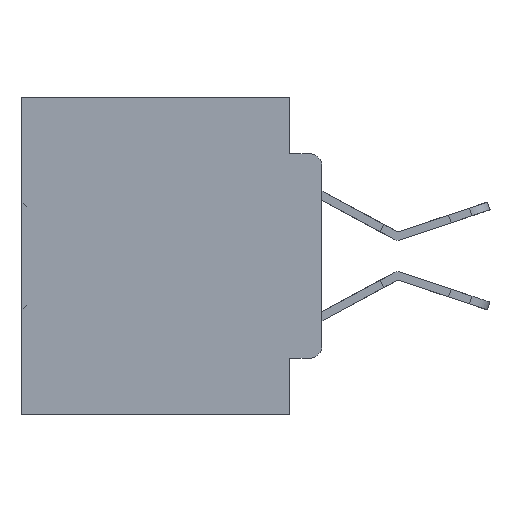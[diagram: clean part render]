
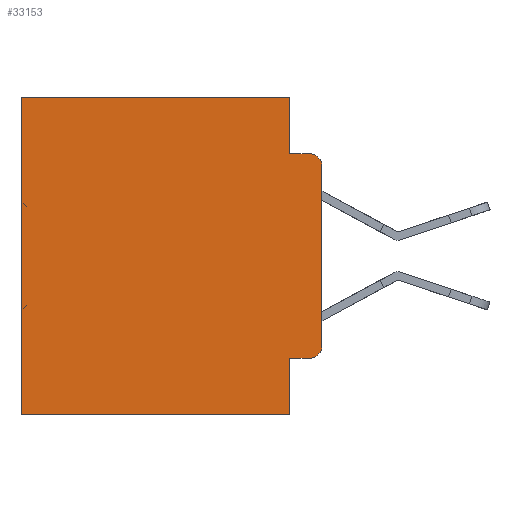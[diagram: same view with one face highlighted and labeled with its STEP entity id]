
A CAD part, left-side view. The second image highlights one B-rep face of the part: STEP entity #33153.
In plain terms, the highlighted planar face has unit normal (-1, 0, 0).
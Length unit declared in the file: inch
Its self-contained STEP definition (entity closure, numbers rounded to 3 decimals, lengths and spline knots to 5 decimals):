
#125 = DIRECTION ( 'NONE',  ( 0., 0., -1. ) ) ;
#1004 = EDGE_CURVE ( 'NONE', #16473, #6473, #36695, .T. ) ;
#1269 = DIRECTION ( 'NONE',  ( 0., 0., -1. ) ) ;
#2205 = PLANE ( 'NONE',  #34444 ) ;
#2926 = CARTESIAN_POINT ( 'NONE',  ( 0.298, 0., 0. ) ) ;
#4104 = DIRECTION ( 'NONE',  ( 0., 0., -1. ) ) ;
#4552 = ORIENTED_EDGE ( 'NONE', *, *, #5437, .T. ) ;
#4838 = CARTESIAN_POINT ( 'NONE',  ( 0.298, 0.051, 0. ) ) ;
#5370 = CARTESIAN_POINT ( 'NONE',  ( 0.298, 0.051, -0.4115 ) ) ;
#5437 = EDGE_CURVE ( 'NONE', #27533, #5798, #13555, .T. ) ;
#5631 = ORIENTED_EDGE ( 'NONE', *, *, #1004, .F. ) ;
#5798 = VERTEX_POINT ( 'NONE', #19166 ) ;
#6473 = VERTEX_POINT ( 'NONE', #28445 ) ;
#6567 = VECTOR ( 'NONE', #1269, 39.37008 ) ;
#7420 = AXIS2_PLACEMENT_3D ( 'NONE', #29748, #24130, #18164 ) ;
#8369 = VECTOR ( 'NONE', #14252, 39.37008 ) ;
#8525 = DIRECTION ( 'NONE',  ( 0., 0., -1. ) ) ;
#8700 = DIRECTION ( 'NONE',  ( -1., 0., 0. ) ) ;
#8850 = ORIENTED_EDGE ( 'NONE', *, *, #24724, .T. ) ;
#9277 = EDGE_CURVE ( 'NONE', #29825, #14734, #18212, .T. ) ;
#9358 = DIRECTION ( 'NONE',  ( 0., 1., 0. ) ) ;
#9427 = CARTESIAN_POINT ( 'NONE',  ( 0.298, 0., -0.3915 ) ) ;
#9529 = EDGE_CURVE ( 'NONE', #6473, #16681, #23020, .T. ) ;
#10790 = LINE ( 'NONE', #4838, #31050 ) ;
#10840 = CARTESIAN_POINT ( 'NONE',  ( 0.298, 0.473, 0. ) ) ;
#10865 = EDGE_CURVE ( 'NONE', #32376, #20447, #12300, .T. ) ;
#10897 = VECTOR ( 'NONE', #33511, 39.37008 ) ;
#11556 = CIRCLE ( 'NONE', #7420, 0.02 ) ;
#11945 = CARTESIAN_POINT ( 'NONE',  ( 0.298, 0.473, -0.5 ) ) ;
#12163 = ORIENTED_EDGE ( 'NONE', *, *, #10865, .T. ) ;
#12300 = LINE ( 'NONE', #32654, #34696 ) ;
#13555 = LINE ( 'NONE', #24939, #27891 ) ;
#14252 = DIRECTION ( 'NONE',  ( 0., -1., 0. ) ) ;
#14734 = VERTEX_POINT ( 'NONE', #9427 ) ;
#15325 = CARTESIAN_POINT ( 'NONE',  ( 0.298, 0., -0.5 ) ) ;
#15423 = CARTESIAN_POINT ( 'NONE',  ( 0.298, 0., 0. ) ) ;
#15704 = VECTOR ( 'NONE', #30556, 39.37008 ) ;
#16250 = ORIENTED_EDGE ( 'NONE', *, *, #9277, .F. ) ;
#16473 = VERTEX_POINT ( 'NONE', #17217 ) ;
#16674 = LINE ( 'NONE', #24885, #10897 ) ;
#16681 = VERTEX_POINT ( 'NONE', #23570 ) ;
#16903 = CARTESIAN_POINT ( 'NONE',  ( 0.298, 0.051, 0. ) ) ;
#17217 = CARTESIAN_POINT ( 'NONE',  ( 0.298, 0.051, 0. ) ) ;
#17577 = ORIENTED_EDGE ( 'NONE', *, *, #19497, .F. ) ;
#18164 = DIRECTION ( 'NONE',  ( 0., 0., -1. ) ) ;
#18212 = LINE ( 'NONE', #15423, #6567 ) ;
#19030 = ORIENTED_EDGE ( 'NONE', *, *, #25948, .T. ) ;
#19166 = CARTESIAN_POINT ( 'NONE',  ( 0.298, 0.02, -0.4115 ) ) ;
#19497 = EDGE_CURVE ( 'NONE', #27533, #29347, #10790, .T. ) ;
#19710 = DIRECTION ( 'NONE',  ( 0., -1., 0. ) ) ;
#19778 = ORIENTED_EDGE ( 'NONE', *, *, #36129, .F. ) ;
#19885 = FACE_OUTER_BOUND ( 'NONE', #29119, .T. ) ;
#19973 = AXIS2_PLACEMENT_3D ( 'NONE', #23063, #8700, #8525 ) ;
#20447 = VERTEX_POINT ( 'NONE', #11945 ) ;
#21294 = ORIENTED_EDGE ( 'NONE', *, *, #9529, .F. ) ;
#23020 = LINE ( 'NONE', #28456, #8369 ) ;
#23063 = CARTESIAN_POINT ( 'NONE',  ( 0.298, 0.02, -0.3915 ) ) ;
#23203 = EDGE_CURVE ( 'NONE', #16473, #32376, #16674, .T. ) ;
#23352 = LINE ( 'NONE', #15325, #23844 ) ;
#23550 = CIRCLE ( 'NONE', #19973, 0.02 ) ;
#23570 = CARTESIAN_POINT ( 'NONE',  ( 0.298, 0.02, -0.0885 ) ) ;
#23844 = VECTOR ( 'NONE', #9358, 39.37008 ) ;
#24130 = DIRECTION ( 'NONE',  ( -1., 0., 0. ) ) ;
#24724 = EDGE_CURVE ( 'NONE', #29825, #16681, #11556, .T. ) ;
#24885 = CARTESIAN_POINT ( 'NONE',  ( 0.298, 0., 0. ) ) ;
#24939 = CARTESIAN_POINT ( 'NONE',  ( 0.298, 0.051, -0.4115 ) ) ;
#25661 = DIRECTION ( 'NONE',  ( 1., 0., 0. ) ) ;
#25948 = EDGE_CURVE ( 'NONE', #5798, #14734, #23550, .T. ) ;
#27533 = VERTEX_POINT ( 'NONE', #5370 ) ;
#27612 = DIRECTION ( 'NONE',  ( 0., 0., -1. ) ) ;
#27891 = VECTOR ( 'NONE', #19710, 39.37008 ) ;
#28445 = CARTESIAN_POINT ( 'NONE',  ( 0.298, 0.051, -0.0885 ) ) ;
#28456 = CARTESIAN_POINT ( 'NONE',  ( 0.298, 0.051, -0.0885 ) ) ;
#29119 = EDGE_LOOP ( 'NONE', ( #16250, #8850, #21294, #5631, #31615, #12163, #19778, #17577, #4552, #19030 ) ) ;
#29347 = VERTEX_POINT ( 'NONE', #33896 ) ;
#29748 = CARTESIAN_POINT ( 'NONE',  ( 0.298, 0.02, -0.1085 ) ) ;
#29825 = VERTEX_POINT ( 'NONE', #31420 ) ;
#30556 = DIRECTION ( 'NONE',  ( 0., 0., -1. ) ) ;
#31050 = VECTOR ( 'NONE', #27612, 39.37008 ) ;
#31420 = CARTESIAN_POINT ( 'NONE',  ( 0.298, 0., -0.1085 ) ) ;
#31615 = ORIENTED_EDGE ( 'NONE', *, *, #23203, .T. ) ;
#32376 = VERTEX_POINT ( 'NONE', #10840 ) ;
#32654 = CARTESIAN_POINT ( 'NONE',  ( 0.298, 0.473, 0. ) ) ;
#33153 = ADVANCED_FACE ( 'NONE', ( #19885 ), #2205, .F. ) ;
#33511 = DIRECTION ( 'NONE',  ( 0., 1., 0. ) ) ;
#33896 = CARTESIAN_POINT ( 'NONE',  ( 0.298, 0.051, -0.5 ) ) ;
#34444 = AXIS2_PLACEMENT_3D ( 'NONE', #2926, #25661, #125 ) ;
#34696 = VECTOR ( 'NONE', #4104, 39.37008 ) ;
#36129 = EDGE_CURVE ( 'NONE', #29347, #20447, #23352, .T. ) ;
#36695 = LINE ( 'NONE', #16903, #15704 ) ;
